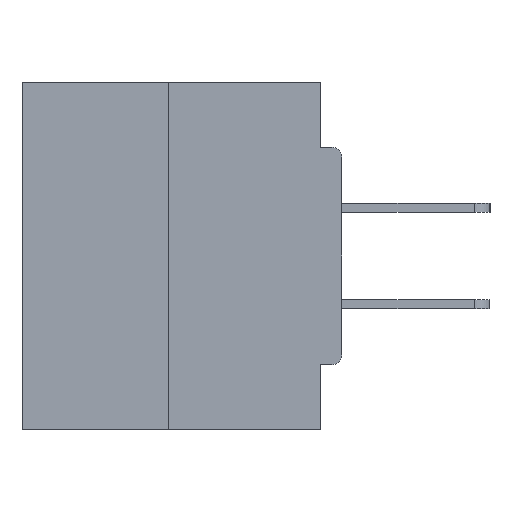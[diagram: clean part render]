
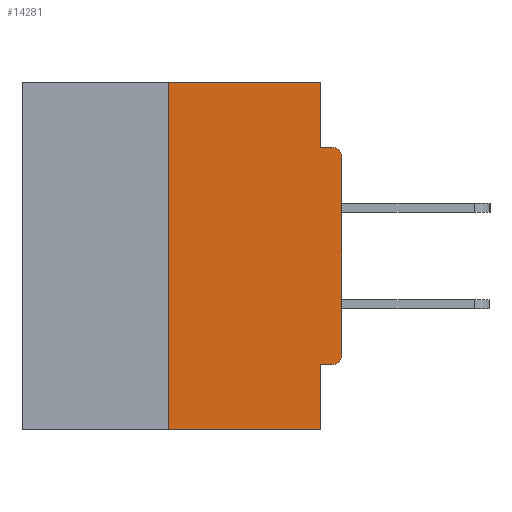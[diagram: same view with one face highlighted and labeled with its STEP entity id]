
A CAD part, left-side view. The second image highlights one B-rep face of the part: STEP entity #14281.
In plain terms, the highlighted planar face has unit normal (-1, 0, 0).
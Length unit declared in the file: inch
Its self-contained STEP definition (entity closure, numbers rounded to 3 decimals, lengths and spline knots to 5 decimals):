
#15 = CARTESIAN_POINT ( 'NONE',  ( 0., 0.46, 0. ) ) ;
#233 = DIRECTION ( 'NONE',  ( 0., 0., -1. ) ) ;
#445 = VECTOR ( 'NONE', #9638, 39.37008 ) ;
#759 = CARTESIAN_POINT ( 'NONE',  ( 0., 0.031, -0.4065 ) ) ;
#1123 = DIRECTION ( 'NONE',  ( 0., -1., 0. ) ) ;
#1253 = LINE ( 'NONE', #21815, #5683 ) ;
#1570 = VERTEX_POINT ( 'NONE', #17615 ) ;
#1780 = EDGE_CURVE ( 'NONE', #18537, #12293, #17988, .T. ) ;
#1816 = LINE ( 'NONE', #14802, #24743 ) ;
#1837 = VERTEX_POINT ( 'NONE', #20855 ) ;
#1841 = VERTEX_POINT ( 'NONE', #28339 ) ;
#1907 = ORIENTED_EDGE ( 'NONE', *, *, #1780, .F. ) ;
#2265 = VERTEX_POINT ( 'NONE', #32451 ) ;
#2639 = VECTOR ( 'NONE', #233, 39.37008 ) ;
#3124 = DIRECTION ( 'NONE',  ( 1., 0., 0. ) ) ;
#3292 = VERTEX_POINT ( 'NONE', #30447 ) ;
#4059 = CARTESIAN_POINT ( 'NONE',  ( 0., 0., -0.0935 ) ) ;
#4088 = CARTESIAN_POINT ( 'NONE',  ( 0., 0.015, -0.1085 ) ) ;
#5683 = VECTOR ( 'NONE', #8951, 39.37008 ) ;
#6377 = VECTOR ( 'NONE', #8250, 39.37008 ) ;
#6394 = ORIENTED_EDGE ( 'NONE', *, *, #32597, .F. ) ;
#6704 = CIRCLE ( 'NONE', #31439, 0.015 ) ;
#7161 = ORIENTED_EDGE ( 'NONE', *, *, #18361, .F. ) ;
#7279 = VERTEX_POINT ( 'NONE', #10739 ) ;
#7477 = ORIENTED_EDGE ( 'NONE', *, *, #15172, .T. ) ;
#7524 = CARTESIAN_POINT ( 'NONE',  ( 0., 0.25, 0. ) ) ;
#7737 = LINE ( 'NONE', #15, #10946 ) ;
#8207 = CARTESIAN_POINT ( 'NONE',  ( 0., 0.015, -0.4065 ) ) ;
#8250 = DIRECTION ( 'NONE',  ( 0., 1., 0. ) ) ;
#8739 = DIRECTION ( 'NONE',  ( 0., -1., 0. ) ) ;
#8817 = ORIENTED_EDGE ( 'NONE', *, *, #23508, .T. ) ;
#8951 = DIRECTION ( 'NONE',  ( 0., 0., -1. ) ) ;
#9638 = DIRECTION ( 'NONE',  ( 0., 0., 1. ) ) ;
#9834 = ORIENTED_EDGE ( 'NONE', *, *, #10093, .T. ) ;
#10093 = EDGE_CURVE ( 'NONE', #1570, #3292, #1816, .T. ) ;
#10343 = DIRECTION ( 'NONE',  ( 0., -1., 0. ) ) ;
#10491 = ORIENTED_EDGE ( 'NONE', *, *, #19257, .T. ) ;
#10495 = DIRECTION ( 'NONE',  ( 0., 0., -1. ) ) ;
#10525 = VECTOR ( 'NONE', #8739, 39.37008 ) ;
#10718 = CARTESIAN_POINT ( 'NONE',  ( 0., 0.46, 0. ) ) ;
#10739 = CARTESIAN_POINT ( 'NONE',  ( 0., 0.25, 0. ) ) ;
#10946 = VECTOR ( 'NONE', #10343, 39.37008 ) ;
#11369 = LINE ( 'NONE', #29577, #10525 ) ;
#11450 = CARTESIAN_POINT ( 'NONE',  ( 0., 0.015, -0.3915 ) ) ;
#11601 = DIRECTION ( 'NONE',  ( 0., 0., -1. ) ) ;
#11825 = EDGE_CURVE ( 'NONE', #2265, #1837, #20215, .T. ) ;
#12293 = VERTEX_POINT ( 'NONE', #30321 ) ;
#12802 = VERTEX_POINT ( 'NONE', #8207 ) ;
#13937 = DIRECTION ( 'NONE',  ( 0., 0., -1. ) ) ;
#14281 = ADVANCED_FACE ( 'NONE', ( #24070 ), #21016, .F. ) ;
#14707 = AXIS2_PLACEMENT_3D ( 'NONE', #10718, #3124, #10495 ) ;
#14802 = CARTESIAN_POINT ( 'NONE',  ( 0., 0., 0. ) ) ;
#15172 = EDGE_CURVE ( 'NONE', #3292, #1837, #6704, .T. ) ;
#15360 = CARTESIAN_POINT ( 'NONE',  ( 0., 0.25, -0.5 ) ) ;
#17103 = DIRECTION ( 'NONE',  ( 0., 0., 1. ) ) ;
#17615 = CARTESIAN_POINT ( 'NONE',  ( 0., 0., -0.3915 ) ) ;
#17859 = AXIS2_PLACEMENT_3D ( 'NONE', #11450, #26516, #13937 ) ;
#17988 = LINE ( 'NONE', #22755, #2639 ) ;
#18361 = EDGE_CURVE ( 'NONE', #28548, #7279, #29805, .T. ) ;
#18537 = VERTEX_POINT ( 'NONE', #759 ) ;
#19257 = EDGE_CURVE ( 'NONE', #12802, #1570, #31713, .T. ) ;
#19974 = EDGE_CURVE ( 'NONE', #12802, #18537, #20077, .T. ) ;
#20077 = LINE ( 'NONE', #26122, #6377 ) ;
#20215 = LINE ( 'NONE', #4059, #31392 ) ;
#20855 = CARTESIAN_POINT ( 'NONE',  ( 0., 0.015, -0.0935 ) ) ;
#21016 = PLANE ( 'NONE',  #14707 ) ;
#21460 = ORIENTED_EDGE ( 'NONE', *, *, #32199, .F. ) ;
#21815 = CARTESIAN_POINT ( 'NONE',  ( 0., 0.031, 0. ) ) ;
#21855 = DIRECTION ( 'NONE',  ( -1., 0., 0. ) ) ;
#22755 = CARTESIAN_POINT ( 'NONE',  ( 0., 0.031, -0.5 ) ) ;
#23508 = EDGE_CURVE ( 'NONE', #28548, #12293, #11369, .T. ) ;
#24070 = FACE_OUTER_BOUND ( 'NONE', #30517, .T. ) ;
#24495 = ORIENTED_EDGE ( 'NONE', *, *, #19974, .F. ) ;
#24743 = VECTOR ( 'NONE', #17103, 39.37008 ) ;
#26122 = CARTESIAN_POINT ( 'NONE',  ( 0., 0., -0.4065 ) ) ;
#26516 = DIRECTION ( 'NONE',  ( -1., 0., 0. ) ) ;
#28339 = CARTESIAN_POINT ( 'NONE',  ( 0., 0.031, 0. ) ) ;
#28548 = VERTEX_POINT ( 'NONE', #15360 ) ;
#28710 = ORIENTED_EDGE ( 'NONE', *, *, #11825, .F. ) ;
#29577 = CARTESIAN_POINT ( 'NONE',  ( 0., 0.46, -0.5 ) ) ;
#29805 = LINE ( 'NONE', #7524, #445 ) ;
#30321 = CARTESIAN_POINT ( 'NONE',  ( 0., 0.031, -0.5 ) ) ;
#30447 = CARTESIAN_POINT ( 'NONE',  ( 0., 0., -0.1085 ) ) ;
#30517 = EDGE_LOOP ( 'NONE', ( #21460, #7161, #8817, #1907, #24495, #10491, #9834, #7477, #28710, #6394 ) ) ;
#31392 = VECTOR ( 'NONE', #1123, 39.37008 ) ;
#31439 = AXIS2_PLACEMENT_3D ( 'NONE', #4088, #21855, #11601 ) ;
#31713 = CIRCLE ( 'NONE', #17859, 0.015 ) ;
#32199 = EDGE_CURVE ( 'NONE', #7279, #1841, #7737, .T. ) ;
#32451 = CARTESIAN_POINT ( 'NONE',  ( 0., 0.031, -0.0935 ) ) ;
#32597 = EDGE_CURVE ( 'NONE', #1841, #2265, #1253, .T. ) ;
